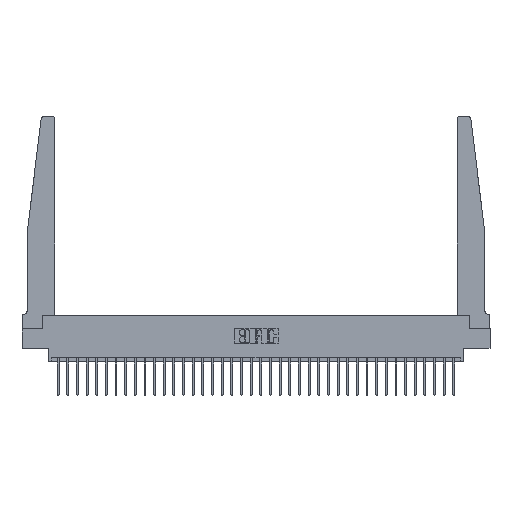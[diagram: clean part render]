
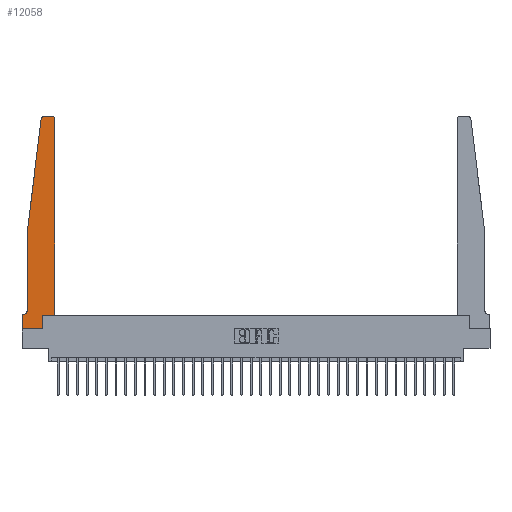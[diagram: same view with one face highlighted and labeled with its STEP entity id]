
A CAD part, top view. The second image highlights one B-rep face of the part: STEP entity #12058.
In plain terms, the highlighted planar face has unit normal (0, 0, 1).
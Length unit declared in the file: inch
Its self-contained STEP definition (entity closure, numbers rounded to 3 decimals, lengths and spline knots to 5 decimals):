
#30 = DIRECTION ( 'NONE',  ( 1., 0., 0. ) ) ;
#475 = CARTESIAN_POINT ( 'NONE',  ( 0.065, 0.2375, 0.37 ) ) ;
#630 = DIRECTION ( 'NONE',  ( 1., 0., 0. ) ) ;
#828 = CARTESIAN_POINT ( 'NONE',  ( 0.395, 2.72, 0.37 ) ) ;
#1298 = LINE ( 'NONE', #8674, #7188 ) ;
#1407 = VERTEX_POINT ( 'NONE', #28750 ) ;
#1519 = DIRECTION ( 'NONE',  ( -1., 0., 0. ) ) ;
#1880 = VERTEX_POINT ( 'NONE', #17954 ) ;
#2081 = VERTEX_POINT ( 'NONE', #3587 ) ;
#2178 = CARTESIAN_POINT ( 'NONE',  ( 0.27653, 2.75, 0.37 ) ) ;
#2205 = ORIENTED_EDGE ( 'NONE', *, *, #3628, .T. ) ;
#2209 = ORIENTED_EDGE ( 'NONE', *, *, #4243, .T. ) ;
#2263 = CARTESIAN_POINT ( 'NONE',  ( 0.425, 2.72, 0.37 ) ) ;
#2646 = LINE ( 'NONE', #28013, #28464 ) ;
#3112 = LINE ( 'NONE', #27490, #15705 ) ;
#3347 = DIRECTION ( 'NONE',  ( 1., 0., 0. ) ) ;
#3587 = CARTESIAN_POINT ( 'NONE',  ( 0.2605, 0., 0.37 ) ) ;
#3628 = EDGE_CURVE ( 'NONE', #27466, #10414, #4623, .T. ) ;
#4228 = DIRECTION ( 'NONE',  ( -1., 0., 0. ) ) ;
#4243 = EDGE_CURVE ( 'NONE', #1407, #1880, #14821, .T. ) ;
#4521 = CARTESIAN_POINT ( 'NONE',  ( 0.24675, 2.72367, 0.37 ) ) ;
#4623 = CIRCLE ( 'NONE', #15142, 0.03 ) ;
#5108 = DIRECTION ( 'NONE',  ( 0., 1., 0. ) ) ;
#5586 = CARTESIAN_POINT ( 'NONE',  ( 0., 0., 0.37 ) ) ;
#6436 = CARTESIAN_POINT ( 'NONE',  ( 0.065, 1.25, 0.37 ) ) ;
#6632 = FACE_OUTER_BOUND ( 'NONE', #8416, .T. ) ;
#7005 = EDGE_CURVE ( 'NONE', #15637, #10732, #28991, .T. ) ;
#7188 = VECTOR ( 'NONE', #13715, 39.37008 ) ;
#7199 = EDGE_CURVE ( 'NONE', #10414, #29768, #11869, .T. ) ;
#7841 = EDGE_CURVE ( 'NONE', #29768, #15637, #20409, .T. ) ;
#7977 = EDGE_CURVE ( 'NONE', #8769, #2081, #3112, .T. ) ;
#8099 = ORIENTED_EDGE ( 'NONE', *, *, #19571, .T. ) ;
#8138 = VECTOR ( 'NONE', #23706, 39.37008 ) ;
#8202 = DIRECTION ( 'NONE',  ( 0., 0., 1. ) ) ;
#8386 = VERTEX_POINT ( 'NONE', #23795 ) ;
#8416 = EDGE_LOOP ( 'NONE', ( #8099, #2205, #10483, #23748, #30337, #31097, #12072, #19450, #20265, #2209, #16349, #10485 ) ) ;
#8674 = CARTESIAN_POINT ( 'NONE',  ( 0.25, 2.75, 0.37 ) ) ;
#8769 = VERTEX_POINT ( 'NONE', #25183 ) ;
#9676 = CARTESIAN_POINT ( 'NONE',  ( 0.065, 1.25, 0.37 ) ) ;
#10414 = VERTEX_POINT ( 'NONE', #4521 ) ;
#10483 = ORIENTED_EDGE ( 'NONE', *, *, #7199, .T. ) ;
#10485 = ORIENTED_EDGE ( 'NONE', *, *, #12098, .T. ) ;
#10732 = VERTEX_POINT ( 'NONE', #30487 ) ;
#11869 = LINE ( 'NONE', #9676, #24332 ) ;
#12058 = ADVANCED_FACE ( 'NONE', ( #6632 ), #30538, .T. ) ;
#12072 = ORIENTED_EDGE ( 'NONE', *, *, #13326, .T. ) ;
#12098 = EDGE_CURVE ( 'NONE', #19894, #8386, #12579, .T. ) ;
#12579 = CIRCLE ( 'NONE', #23030, 0.03 ) ;
#12718 = EDGE_CURVE ( 'NONE', #1880, #19894, #2646, .T. ) ;
#13326 = EDGE_CURVE ( 'NONE', #28793, #8769, #18701, .T. ) ;
#13715 = DIRECTION ( 'NONE',  ( -1., 0., 0. ) ) ;
#14821 = LINE ( 'NONE', #26115, #8138 ) ;
#15142 = AXIS2_PLACEMENT_3D ( 'NONE', #30565, #15692, #630 ) ;
#15633 = DIRECTION ( 'NONE',  ( 0., 1., 0. ) ) ;
#15637 = VERTEX_POINT ( 'NONE', #475 ) ;
#15692 = DIRECTION ( 'NONE',  ( 0., 0., 1. ) ) ;
#15705 = VECTOR ( 'NONE', #30, 39.37008 ) ;
#16349 = ORIENTED_EDGE ( 'NONE', *, *, #12718, .T. ) ;
#16553 = DIRECTION ( 'NONE',  ( 0., 0., -1. ) ) ;
#17039 = DIRECTION ( 'NONE',  ( 0., -1., 0. ) ) ;
#17918 = VECTOR ( 'NONE', #30569, 39.37008 ) ;
#17954 = CARTESIAN_POINT ( 'NONE',  ( 0.425, 0.18, 0.37 ) ) ;
#18364 = DIRECTION ( 'NONE',  ( 0., 0., 1. ) ) ;
#18701 = LINE ( 'NONE', #5586, #17918 ) ;
#19450 = ORIENTED_EDGE ( 'NONE', *, *, #7977, .T. ) ;
#19571 = EDGE_CURVE ( 'NONE', #8386, #27466, #1298, .T. ) ;
#19610 = VECTOR ( 'NONE', #17039, 39.37008 ) ;
#19894 = VERTEX_POINT ( 'NONE', #2263 ) ;
#20017 = EDGE_CURVE ( 'NONE', #2081, #1407, #28637, .T. ) ;
#20265 = ORIENTED_EDGE ( 'NONE', *, *, #20017, .T. ) ;
#20409 = LINE ( 'NONE', #26961, #19610 ) ;
#21067 = EDGE_CURVE ( 'NONE', #10732, #28793, #24706, .T. ) ;
#21361 = AXIS2_PLACEMENT_3D ( 'NONE', #23187, #8202, #25687 ) ;
#22700 = CARTESIAN_POINT ( 'NONE',  ( 0., 0.1875, 0.37 ) ) ;
#23030 = AXIS2_PLACEMENT_3D ( 'NONE', #828, #18364, #3347 ) ;
#23187 = CARTESIAN_POINT ( 'NONE',  ( 0., 0.1875, 0.37 ) ) ;
#23706 = DIRECTION ( 'NONE',  ( 1., 0., 0. ) ) ;
#23748 = ORIENTED_EDGE ( 'NONE', *, *, #7841, .T. ) ;
#23795 = CARTESIAN_POINT ( 'NONE',  ( 0.395, 2.75, 0.37 ) ) ;
#23916 = VECTOR ( 'NONE', #4228, 39.37008 ) ;
#24278 = CARTESIAN_POINT ( 'NONE',  ( 0.065, 0.1875, 0.37 ) ) ;
#24332 = VECTOR ( 'NONE', #27104, 39.37008 ) ;
#24706 = LINE ( 'NONE', #24278, #23916 ) ;
#25183 = CARTESIAN_POINT ( 'NONE',  ( 0., 0., 0.37 ) ) ;
#25687 = DIRECTION ( 'NONE',  ( 1., 0., 0. ) ) ;
#26115 = CARTESIAN_POINT ( 'NONE',  ( 0.425, 0.18, 0.37 ) ) ;
#26961 = CARTESIAN_POINT ( 'NONE',  ( 0.065, 1.25, 0.37 ) ) ;
#27104 = DIRECTION ( 'NONE',  ( -0.122, -0.992, 0. ) ) ;
#27466 = VERTEX_POINT ( 'NONE', #2178 ) ;
#27490 = CARTESIAN_POINT ( 'NONE',  ( 0., 0., 0.37 ) ) ;
#27866 = VECTOR ( 'NONE', #5108, 39.37008 ) ;
#28013 = CARTESIAN_POINT ( 'NONE',  ( 0.425, 0.18, 0.37 ) ) ;
#28332 = AXIS2_PLACEMENT_3D ( 'NONE', #31430, #16553, #1519 ) ;
#28464 = VECTOR ( 'NONE', #15633, 39.37008 ) ;
#28637 = LINE ( 'NONE', #29997, #27866 ) ;
#28750 = CARTESIAN_POINT ( 'NONE',  ( 0.2605, 0.18, 0.37 ) ) ;
#28793 = VERTEX_POINT ( 'NONE', #22700 ) ;
#28991 = CIRCLE ( 'NONE', #28332, 0.05 ) ;
#29768 = VERTEX_POINT ( 'NONE', #6436 ) ;
#29997 = CARTESIAN_POINT ( 'NONE',  ( 0.2605, 0.18, 0.37 ) ) ;
#30337 = ORIENTED_EDGE ( 'NONE', *, *, #7005, .T. ) ;
#30487 = CARTESIAN_POINT ( 'NONE',  ( 0.015, 0.1875, 0.37 ) ) ;
#30538 = PLANE ( 'NONE',  #21361 ) ;
#30565 = CARTESIAN_POINT ( 'NONE',  ( 0.27653, 2.72, 0.37 ) ) ;
#30569 = DIRECTION ( 'NONE',  ( 0., -1., 0. ) ) ;
#31097 = ORIENTED_EDGE ( 'NONE', *, *, #21067, .T. ) ;
#31430 = CARTESIAN_POINT ( 'NONE',  ( 0.015, 0.2375, 0.37 ) ) ;
